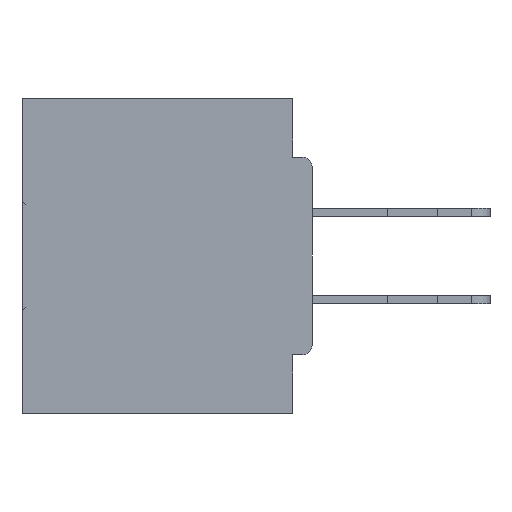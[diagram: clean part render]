
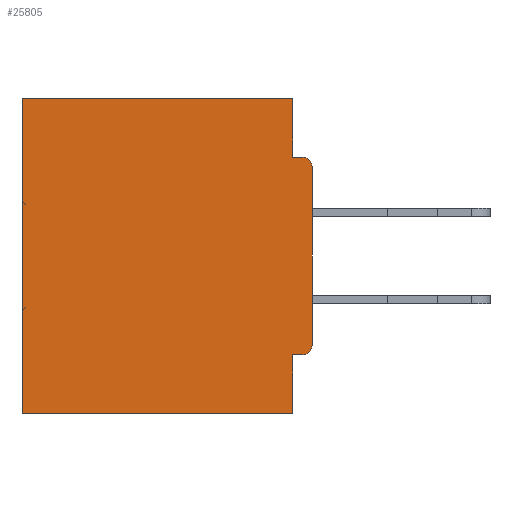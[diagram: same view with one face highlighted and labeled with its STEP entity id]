
A CAD part, left-side view. The second image highlights one B-rep face of the part: STEP entity #25805.
In plain terms, the highlighted planar face has unit normal (-1, 0, 0).
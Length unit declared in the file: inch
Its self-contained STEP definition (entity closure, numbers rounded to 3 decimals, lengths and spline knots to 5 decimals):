
#1054 = DIRECTION ( 'NONE',  ( -1., 0., 0. ) ) ;
#1164 = DIRECTION ( 'NONE',  ( 0., 0., -1. ) ) ;
#1234 = ORIENTED_EDGE ( 'NONE', *, *, #6593, .T. ) ;
#2405 = DIRECTION ( 'NONE',  ( 0., 0., -1. ) ) ;
#2831 = DIRECTION ( 'NONE',  ( 0., 0., -1. ) ) ;
#3239 = EDGE_CURVE ( 'NONE', #17129, #42106, #7929, .T. ) ;
#3706 = EDGE_CURVE ( 'NONE', #42106, #36943, #14522, .T. ) ;
#5100 = VECTOR ( 'NONE', #34116, 39.37008 ) ;
#6593 = EDGE_CURVE ( 'NONE', #19236, #30686, #38324, .T. ) ;
#7729 = FACE_OUTER_BOUND ( 'NONE', #32436, .T. ) ;
#7921 = VERTEX_POINT ( 'NONE', #31576 ) ;
#7929 = LINE ( 'NONE', #43291, #35838 ) ;
#8058 = DIRECTION ( 'NONE',  ( 0., 0., -1. ) ) ;
#8832 = AXIS2_PLACEMENT_3D ( 'NONE', #34770, #16876, #2831 ) ;
#9027 = ORIENTED_EDGE ( 'NONE', *, *, #18458, .F. ) ;
#9333 = VERTEX_POINT ( 'NONE', #34354 ) ;
#9670 = LINE ( 'NONE', #19897, #15693 ) ;
#11355 = EDGE_CURVE ( 'NONE', #19236, #9333, #9670, .T. ) ;
#11749 = CARTESIAN_POINT ( 'NONE',  ( 0.298, 0.015, -0.3915 ) ) ;
#13665 = VECTOR ( 'NONE', #20986, 39.37008 ) ;
#13714 = CARTESIAN_POINT ( 'NONE',  ( 0.298, 0.46, -0.5 ) ) ;
#13785 = VECTOR ( 'NONE', #27123, 39.37008 ) ;
#13982 = VERTEX_POINT ( 'NONE', #33409 ) ;
#14522 = LINE ( 'NONE', #36744, #5100 ) ;
#15693 = VECTOR ( 'NONE', #2405, 39.37008 ) ;
#16296 = CARTESIAN_POINT ( 'NONE',  ( 0.298, 0.031, -0.5 ) ) ;
#16367 = EDGE_CURVE ( 'NONE', #13982, #7921, #26394, .T. ) ;
#16876 = DIRECTION ( 'NONE',  ( -1., 0., 0. ) ) ;
#17129 = VERTEX_POINT ( 'NONE', #34592 ) ;
#18458 = EDGE_CURVE ( 'NONE', #36788, #30686, #31554, .T. ) ;
#19008 = AXIS2_PLACEMENT_3D ( 'NONE', #11749, #1054, #8058 ) ;
#19215 = AXIS2_PLACEMENT_3D ( 'NONE', #32932, #21663, #39792 ) ;
#19236 = VERTEX_POINT ( 'NONE', #33577 ) ;
#19897 = CARTESIAN_POINT ( 'NONE',  ( 0.298, 0., 0. ) ) ;
#20925 = VERTEX_POINT ( 'NONE', #24165 ) ;
#20986 = DIRECTION ( 'NONE',  ( 0., -1., 0. ) ) ;
#21048 = LINE ( 'NONE', #23705, #21580 ) ;
#21580 = VECTOR ( 'NONE', #41540, 39.37008 ) ;
#21663 = DIRECTION ( 'NONE',  ( 1., 0., 0. ) ) ;
#22094 = ORIENTED_EDGE ( 'NONE', *, *, #3706, .F. ) ;
#22111 = CARTESIAN_POINT ( 'NONE',  ( 0.298, 0.031, -0.0935 ) ) ;
#22112 = PLANE ( 'NONE',  #19215 ) ;
#23021 = VECTOR ( 'NONE', #1164, 39.37008 ) ;
#23705 = CARTESIAN_POINT ( 'NONE',  ( 0.298, 0., -0.4065 ) ) ;
#23973 = ORIENTED_EDGE ( 'NONE', *, *, #26255, .F. ) ;
#24165 = CARTESIAN_POINT ( 'NONE',  ( 0.298, 0.015, -0.4065 ) ) ;
#24928 = CARTESIAN_POINT ( 'NONE',  ( 0.298, 0., -0.0935 ) ) ;
#25805 = ADVANCED_FACE ( 'NONE', ( #7729 ), #22112, .F. ) ;
#26054 = LINE ( 'NONE', #34627, #13785 ) ;
#26255 = EDGE_CURVE ( 'NONE', #13982, #36788, #26054, .T. ) ;
#26362 = ORIENTED_EDGE ( 'NONE', *, *, #41245, .T. ) ;
#26394 = LINE ( 'NONE', #35093, #38708 ) ;
#27123 = DIRECTION ( 'NONE',  ( 0., 0., -1. ) ) ;
#29202 = CARTESIAN_POINT ( 'NONE',  ( 0.298, 0.46, 0. ) ) ;
#30686 = VERTEX_POINT ( 'NONE', #41930 ) ;
#31171 = ORIENTED_EDGE ( 'NONE', *, *, #46103, .F. ) ;
#31554 = LINE ( 'NONE', #24928, #13665 ) ;
#31576 = CARTESIAN_POINT ( 'NONE',  ( 0.298, 0.46, 0. ) ) ;
#32436 = EDGE_LOOP ( 'NONE', ( #1234, #9027, #23973, #33176, #26362, #22094, #36295, #31171, #45158, #39552 ) ) ;
#32563 = LINE ( 'NONE', #29202, #23021 ) ;
#32932 = CARTESIAN_POINT ( 'NONE',  ( 0.298, 0., 0. ) ) ;
#33176 = ORIENTED_EDGE ( 'NONE', *, *, #16367, .T. ) ;
#33409 = CARTESIAN_POINT ( 'NONE',  ( 0.298, 0.031, 0. ) ) ;
#33577 = CARTESIAN_POINT ( 'NONE',  ( 0.298, 0., -0.1085 ) ) ;
#34116 = DIRECTION ( 'NONE',  ( 0., 1., 0. ) ) ;
#34354 = CARTESIAN_POINT ( 'NONE',  ( 0.298, 0., -0.3915 ) ) ;
#34592 = CARTESIAN_POINT ( 'NONE',  ( 0.298, 0.031, -0.4065 ) ) ;
#34627 = CARTESIAN_POINT ( 'NONE',  ( 0.298, 0.031, -0.5 ) ) ;
#34770 = CARTESIAN_POINT ( 'NONE',  ( 0.298, 0.015, -0.1085 ) ) ;
#35093 = CARTESIAN_POINT ( 'NONE',  ( 0.298, 0., 0. ) ) ;
#35570 = CIRCLE ( 'NONE', #19008, 0.015 ) ;
#35838 = VECTOR ( 'NONE', #39427, 39.37008 ) ;
#36295 = ORIENTED_EDGE ( 'NONE', *, *, #3239, .F. ) ;
#36744 = CARTESIAN_POINT ( 'NONE',  ( 0.298, 0., -0.5 ) ) ;
#36788 = VERTEX_POINT ( 'NONE', #22111 ) ;
#36943 = VERTEX_POINT ( 'NONE', #13714 ) ;
#38324 = CIRCLE ( 'NONE', #8832, 0.015 ) ;
#38708 = VECTOR ( 'NONE', #41793, 39.37008 ) ;
#39080 = EDGE_CURVE ( 'NONE', #20925, #9333, #35570, .T. ) ;
#39427 = DIRECTION ( 'NONE',  ( 0., 0., -1. ) ) ;
#39552 = ORIENTED_EDGE ( 'NONE', *, *, #11355, .F. ) ;
#39792 = DIRECTION ( 'NONE',  ( 0., 0., -1. ) ) ;
#41245 = EDGE_CURVE ( 'NONE', #7921, #36943, #32563, .T. ) ;
#41540 = DIRECTION ( 'NONE',  ( 0., 1., 0. ) ) ;
#41793 = DIRECTION ( 'NONE',  ( 0., 1., 0. ) ) ;
#41930 = CARTESIAN_POINT ( 'NONE',  ( 0.298, 0.015, -0.0935 ) ) ;
#42106 = VERTEX_POINT ( 'NONE', #16296 ) ;
#43291 = CARTESIAN_POINT ( 'NONE',  ( 0.298, 0.031, -0.5 ) ) ;
#45158 = ORIENTED_EDGE ( 'NONE', *, *, #39080, .T. ) ;
#46103 = EDGE_CURVE ( 'NONE', #20925, #17129, #21048, .T. ) ;
